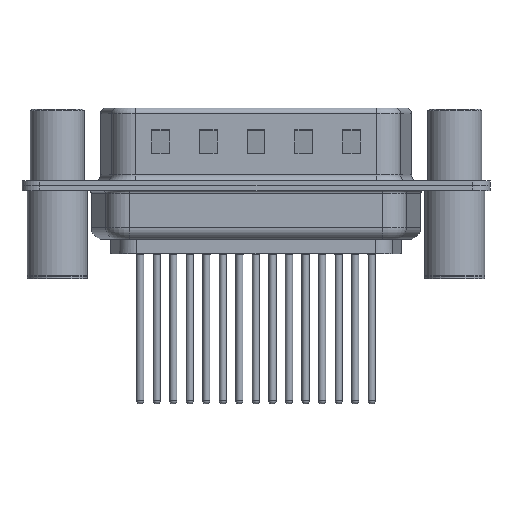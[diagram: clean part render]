
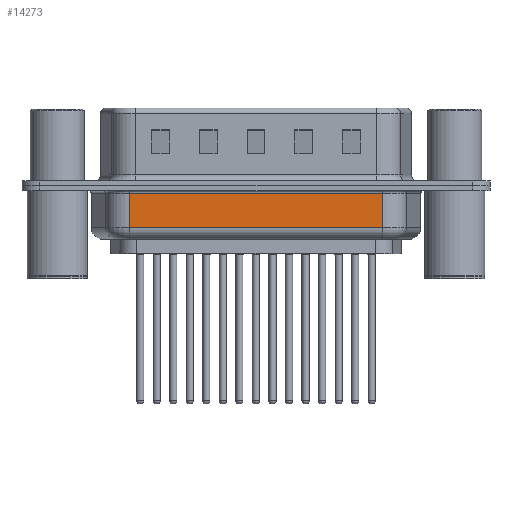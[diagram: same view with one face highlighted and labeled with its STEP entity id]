
A CAD part, front view. The second image highlights one B-rep face of the part: STEP entity #14273.
In plain terms, the highlighted planar face has unit normal (0, -1, 0).
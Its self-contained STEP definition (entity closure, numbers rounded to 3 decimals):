
#331 = VERTEX_POINT ( 'NONE', #8622 ) ;
#825 = CARTESIAN_POINT ( 'NONE',  ( 6.031, -5.35, -0.65 ) ) ;
#2791 = LINE ( 'NONE', #6969, #6514 ) ;
#3050 = VECTOR ( 'NONE', #8650, 1000. ) ;
#3433 = EDGE_CURVE ( 'NONE', #10945, #11520, #2791, .T. ) ;
#3626 = FACE_OUTER_BOUND ( 'NONE', #17604, .T. ) ;
#4186 = ORIENTED_EDGE ( 'NONE', *, *, #11891, .F. ) ;
#4605 = EDGE_CURVE ( 'NONE', #9895, #10945, #10805, .T. ) ;
#5011 = DIRECTION ( 'NONE',  ( -1., 0., 0. ) ) ;
#6224 = CARTESIAN_POINT ( 'NONE',  ( 27.269, -5.35, -3.5 ) ) ;
#6514 = VECTOR ( 'NONE', #18384, 1000. ) ;
#6669 = PLANE ( 'NONE',  #12665 ) ;
#6969 = CARTESIAN_POINT ( 'NONE',  ( 27.269, -5.35, -4.5 ) ) ;
#7971 = DIRECTION ( 'NONE',  ( 1., 0., 0. ) ) ;
#8567 = CARTESIAN_POINT ( 'NONE',  ( 6.031, -5.35, -4.5 ) ) ;
#8622 = CARTESIAN_POINT ( 'NONE',  ( 6.031, -5.35, -0.65 ) ) ;
#8650 = DIRECTION ( 'NONE',  ( 0., 0., 1. ) ) ;
#9895 = VERTEX_POINT ( 'NONE', #10936 ) ;
#10178 = EDGE_CURVE ( 'NONE', #11520, #331, #13839, .T. ) ;
#10199 = ORIENTED_EDGE ( 'NONE', *, *, #10178, .T. ) ;
#10805 = LINE ( 'NONE', #15194, #15005 ) ;
#10936 = CARTESIAN_POINT ( 'NONE',  ( 6.031, -5.35, -3.5 ) ) ;
#10945 = VERTEX_POINT ( 'NONE', #6224 ) ;
#11261 = ORIENTED_EDGE ( 'NONE', *, *, #3433, .T. ) ;
#11520 = VERTEX_POINT ( 'NONE', #15992 ) ;
#11891 = EDGE_CURVE ( 'NONE', #9895, #331, #16777, .T. ) ;
#12045 = ORIENTED_EDGE ( 'NONE', *, *, #4605, .T. ) ;
#12268 = CARTESIAN_POINT ( 'NONE',  ( 6.031, -5.35, -4.5 ) ) ;
#12450 = DIRECTION ( 'NONE',  ( -1., 0., 0. ) ) ;
#12665 = AXIS2_PLACEMENT_3D ( 'NONE', #12268, #18005, #12450 ) ;
#13605 = VECTOR ( 'NONE', #5011, 1000. ) ;
#13839 = LINE ( 'NONE', #825, #13605 ) ;
#14273 = ADVANCED_FACE ( 'NONE', ( #3626 ), #6669, .F. ) ;
#15005 = VECTOR ( 'NONE', #7971, 1000. ) ;
#15194 = CARTESIAN_POINT ( 'NONE',  ( 6.031, -5.35, -3.5 ) ) ;
#15992 = CARTESIAN_POINT ( 'NONE',  ( 27.269, -5.35, -0.65 ) ) ;
#16777 = LINE ( 'NONE', #8567, #3050 ) ;
#17604 = EDGE_LOOP ( 'NONE', ( #4186, #12045, #11261, #10199 ) ) ;
#18005 = DIRECTION ( 'NONE',  ( 0., 1., 0. ) ) ;
#18384 = DIRECTION ( 'NONE',  ( 0., 0., 1. ) ) ;
